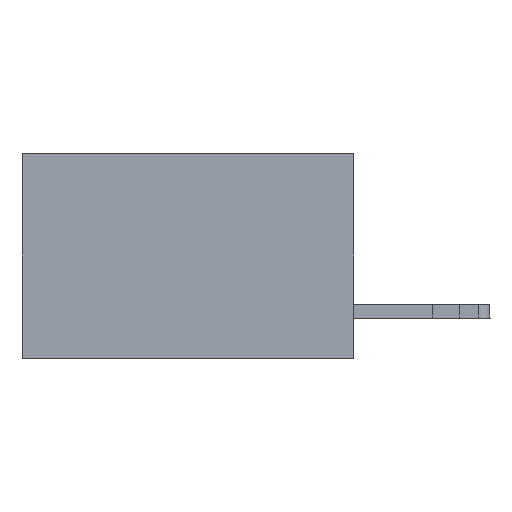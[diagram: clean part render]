
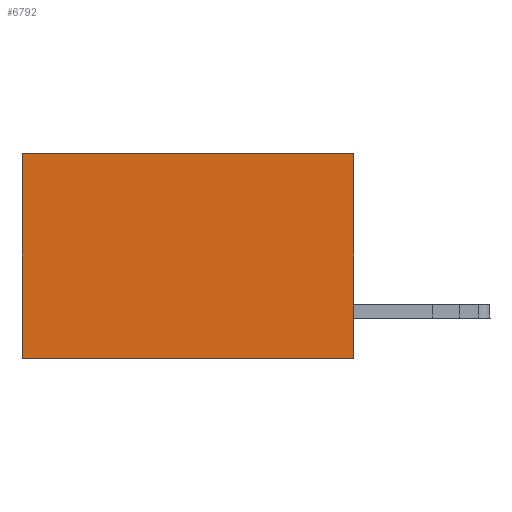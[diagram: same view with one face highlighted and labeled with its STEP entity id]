
A CAD part, left-side view. The second image highlights one B-rep face of the part: STEP entity #6792.
In plain terms, the highlighted planar face has unit normal (-1, 0, 0).
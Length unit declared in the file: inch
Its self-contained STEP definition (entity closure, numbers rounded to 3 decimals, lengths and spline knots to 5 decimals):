
#177 = VECTOR ( 'NONE', #8790, 39.37008 ) ;
#604 = CARTESIAN_POINT ( 'NONE',  ( 0.2875, 0., 0. ) ) ;
#1210 = LINE ( 'NONE', #604, #9323 ) ;
#2168 = VERTEX_POINT ( 'NONE', #17712 ) ;
#2540 = EDGE_LOOP ( 'NONE', ( #22741, #9563, #21523, #5496 ) ) ;
#2981 = VERTEX_POINT ( 'NONE', #8637 ) ;
#3380 = CARTESIAN_POINT ( 'NONE',  ( 0.2875, 0., 0. ) ) ;
#4278 = CARTESIAN_POINT ( 'NONE',  ( 0.2875, 0.6, 0. ) ) ;
#5051 = LINE ( 'NONE', #4278, #18738 ) ;
#5114 = CARTESIAN_POINT ( 'NONE',  ( 0.2875, 0.6, 0. ) ) ;
#5496 = ORIENTED_EDGE ( 'NONE', *, *, #22969, .T. ) ;
#5990 = DIRECTION ( 'NONE',  ( 0., 0., -1. ) ) ;
#6792 = ADVANCED_FACE ( 'NONE', ( #13761 ), #7812, .F. ) ;
#7030 = EDGE_CURVE ( 'NONE', #20758, #2168, #18446, .T. ) ;
#7812 = PLANE ( 'NONE',  #11199 ) ;
#8052 = CARTESIAN_POINT ( 'NONE',  ( 0.2875, 0., 0. ) ) ;
#8298 = DIRECTION ( 'NONE',  ( 1., 0., 0. ) ) ;
#8637 = CARTESIAN_POINT ( 'NONE',  ( 0.2875, 0., 0. ) ) ;
#8790 = DIRECTION ( 'NONE',  ( 0., 1., 0. ) ) ;
#9323 = VECTOR ( 'NONE', #5990, 39.37008 ) ;
#9563 = ORIENTED_EDGE ( 'NONE', *, *, #7030, .F. ) ;
#10787 = VERTEX_POINT ( 'NONE', #5114 ) ;
#11199 = AXIS2_PLACEMENT_3D ( 'NONE', #8052, #8298, #17845 ) ;
#11255 = CARTESIAN_POINT ( 'NONE',  ( 0.2875, 0., -0.37 ) ) ;
#13761 = FACE_OUTER_BOUND ( 'NONE', #2540, .T. ) ;
#14033 = VECTOR ( 'NONE', #18528, 39.37008 ) ;
#14355 = EDGE_CURVE ( 'NONE', #10787, #2168, #5051, .T. ) ;
#14461 = CARTESIAN_POINT ( 'NONE',  ( 0.2875, 0., -0.37 ) ) ;
#17712 = CARTESIAN_POINT ( 'NONE',  ( 0.2875, 0.6, -0.37 ) ) ;
#17845 = DIRECTION ( 'NONE',  ( 0., 0., -1. ) ) ;
#18446 = LINE ( 'NONE', #11255, #14033 ) ;
#18528 = DIRECTION ( 'NONE',  ( 0., 1., 0. ) ) ;
#18738 = VECTOR ( 'NONE', #20820, 39.37008 ) ;
#19804 = LINE ( 'NONE', #3380, #177 ) ;
#20122 = EDGE_CURVE ( 'NONE', #2981, #20758, #1210, .T. ) ;
#20758 = VERTEX_POINT ( 'NONE', #14461 ) ;
#20820 = DIRECTION ( 'NONE',  ( 0., 0., -1. ) ) ;
#21523 = ORIENTED_EDGE ( 'NONE', *, *, #20122, .F. ) ;
#22741 = ORIENTED_EDGE ( 'NONE', *, *, #14355, .T. ) ;
#22969 = EDGE_CURVE ( 'NONE', #2981, #10787, #19804, .T. ) ;
